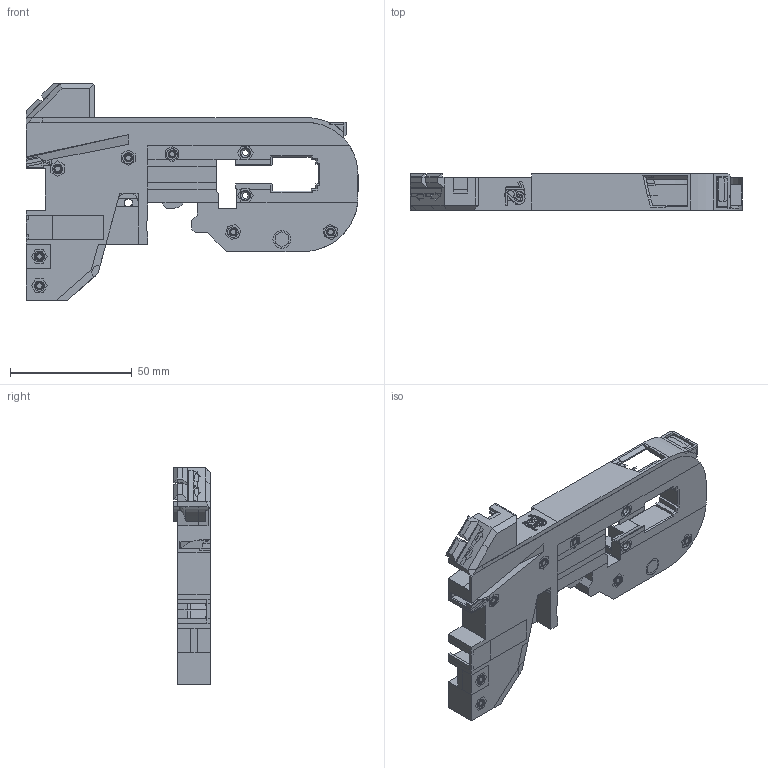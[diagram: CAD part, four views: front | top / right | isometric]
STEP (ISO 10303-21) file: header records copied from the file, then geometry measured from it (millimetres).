
FILE_DESCRIPTION(('FreeCAD Model'),'2;1');
FILE_NAME('Open CASCADE Shape Model','2025-01-14T14:45:39',(''),(''), 'Open CASCADE STEP processor 7.6','FreeCAD','Unknown');
FILE_SCHEMA(('AUTOMOTIVE_DESIGN { 1 0 10303 214 1 1 1 1 }'));
Length unit declared in the file: millimetre
Products named in the file (1): Body001
Bounding box: 136.25 x 15 x 88.9 mm (x, y, z)
Volume: 58555.1 mm3; surface area: 31091.5 mm2
Topology: 7 solids, 7 shells, 1055 faces, 3118 edges, 2138 vertices
Faces by surface type: plane 774, bspline 198, cylinder 41, extrusion 31, cone 10, revolution 1
Full cylindrical faces by diameter (mm): 2.25 x7, 2.45 x2, 3.2 x1, 7 x1
Entity records: 47009 total; most frequent: CARTESIAN_POINT 12515, ORIENTED_EDGE 6234, DIRECTION 4636, EDGE_CURVE 3116, VERTEX_POINT 2138, VECTOR 2107, LINE 2076, AXIS2_PLACEMENT_3D 1264
